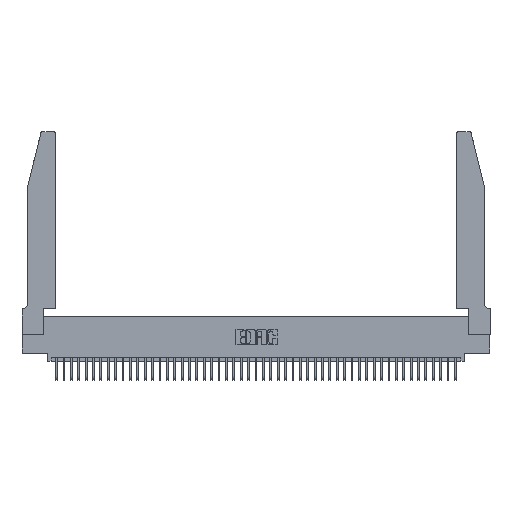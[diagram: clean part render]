
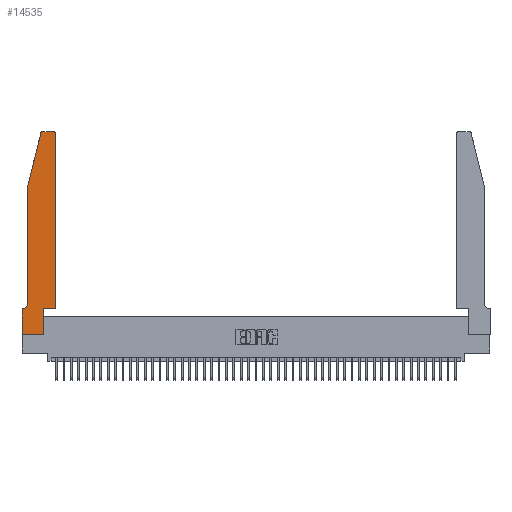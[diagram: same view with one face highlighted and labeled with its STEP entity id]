
A CAD part, top view. The second image highlights one B-rep face of the part: STEP entity #14535.
In plain terms, the highlighted planar face has unit normal (0, 0, 1).
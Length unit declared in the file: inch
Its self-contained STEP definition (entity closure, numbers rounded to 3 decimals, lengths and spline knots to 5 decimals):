
#66 = CARTESIAN_POINT ( 'NONE',  ( 0.2865, 0.35, 0.37 ) ) ;
#207 = VECTOR ( 'NONE', #40731, 39.37008 ) ;
#488 = CARTESIAN_POINT ( 'NONE',  ( 0., 0., 0.37 ) ) ;
#672 = CARTESIAN_POINT ( 'NONE',  ( 0.25487, 2.72718, 0.37 ) ) ;
#679 = VERTEX_POINT ( 'NONE', #22662 ) ;
#1018 = CARTESIAN_POINT ( 'NONE',  ( 0.4505, 0.35, 0.37 ) ) ;
#1709 = ORIENTED_EDGE ( 'NONE', *, *, #38244, .T. ) ;
#1734 = VECTOR ( 'NONE', #15758, 39.37008 ) ;
#2742 = DIRECTION ( 'NONE',  ( 0., 0., -1. ) ) ;
#3616 = CARTESIAN_POINT ( 'NONE',  ( 0.4505, 2.72, 0.37 ) ) ;
#4556 = DIRECTION ( 'NONE',  ( 1., 0., 0. ) ) ;
#5175 = ORIENTED_EDGE ( 'NONE', *, *, #9305, .T. ) ;
#5459 = LINE ( 'NONE', #34822, #13604 ) ;
#5565 = EDGE_CURVE ( 'NONE', #23691, #679, #12324, .T. ) ;
#5816 = ORIENTED_EDGE ( 'NONE', *, *, #7570, .T. ) ;
#6115 = VECTOR ( 'NONE', #41882, 39.37008 ) ;
#6336 = DIRECTION ( 'NONE',  ( 0., 0., 1. ) ) ;
#7570 = EDGE_CURVE ( 'NONE', #679, #35462, #41618, .T. ) ;
#8010 = DIRECTION ( 'NONE',  ( 0., 0., 1. ) ) ;
#8549 = VECTOR ( 'NONE', #20804, 39.37008 ) ;
#8889 = CARTESIAN_POINT ( 'NONE',  ( 0., 0., 0.37 ) ) ;
#9305 = EDGE_CURVE ( 'NONE', #35161, #23691, #12221, .T. ) ;
#9430 = VERTEX_POINT ( 'NONE', #10412 ) ;
#9630 = DIRECTION ( 'NONE',  ( -1., 0., 0. ) ) ;
#10412 = CARTESIAN_POINT ( 'NONE',  ( 0.4205, 2.75, 0.37 ) ) ;
#10415 = CIRCLE ( 'NONE', #20290, 0.03 ) ;
#10791 = EDGE_CURVE ( 'NONE', #35462, #15622, #33499, .T. ) ;
#10828 = PLANE ( 'NONE',  #28734 ) ;
#12221 = CIRCLE ( 'NONE', #22729, 0.07 ) ;
#12324 = LINE ( 'NONE', #30077, #20281 ) ;
#12416 = CARTESIAN_POINT ( 'NONE',  ( 0.0755, 2., 0.37 ) ) ;
#12684 = LINE ( 'NONE', #12416, #29736 ) ;
#13153 = VERTEX_POINT ( 'NONE', #42858 ) ;
#13346 = CARTESIAN_POINT ( 'NONE',  ( 0.0755, 2., 0.37 ) ) ;
#13604 = VECTOR ( 'NONE', #17772, 39.37008 ) ;
#13966 = CIRCLE ( 'NONE', #28498, 0.03 ) ;
#14257 = DIRECTION ( 'NONE',  ( 0., 0., 1. ) ) ;
#14535 = ADVANCED_FACE ( 'NONE', ( #36856 ), #10828, .T. ) ;
#14954 = EDGE_CURVE ( 'NONE', #28497, #17922, #13966, .T. ) ;
#15125 = ORIENTED_EDGE ( 'NONE', *, *, #26825, .T. ) ;
#15622 = VERTEX_POINT ( 'NONE', #16986 ) ;
#15758 = DIRECTION ( 'NONE',  ( 0., 1., 0. ) ) ;
#16553 = ORIENTED_EDGE ( 'NONE', *, *, #17469, .T. ) ;
#16986 = CARTESIAN_POINT ( 'NONE',  ( 0.2865, 0., 0.37 ) ) ;
#17469 = EDGE_CURVE ( 'NONE', #13153, #20278, #30271, .T. ) ;
#17772 = DIRECTION ( 'NONE',  ( -1., 0., 0. ) ) ;
#17922 = VERTEX_POINT ( 'NONE', #672 ) ;
#19281 = EDGE_CURVE ( 'NONE', #43504, #13153, #43596, .T. ) ;
#20278 = VERTEX_POINT ( 'NONE', #3616 ) ;
#20281 = VECTOR ( 'NONE', #9630, 39.37008 ) ;
#20290 = AXIS2_PLACEMENT_3D ( 'NONE', #28475, #8010, #31989 ) ;
#20804 = DIRECTION ( 'NONE',  ( 0., 1., 0. ) ) ;
#21952 = ORIENTED_EDGE ( 'NONE', *, *, #14954, .T. ) ;
#22313 = VECTOR ( 'NONE', #36286, 39.37008 ) ;
#22662 = CARTESIAN_POINT ( 'NONE',  ( 0., 0.35, 0.37 ) ) ;
#22723 = EDGE_CURVE ( 'NONE', #9430, #28497, #5459, .T. ) ;
#22729 = AXIS2_PLACEMENT_3D ( 'NONE', #23378, #2742, #26778 ) ;
#23218 = EDGE_LOOP ( 'NONE', ( #23835, #21952, #43551, #15125, #5175, #38683, #5816, #31311, #1709, #23413, #16553, #39339 ) ) ;
#23378 = CARTESIAN_POINT ( 'NONE',  ( 0.0055, 0.42, 0.37 ) ) ;
#23413 = ORIENTED_EDGE ( 'NONE', *, *, #19281, .T. ) ;
#23691 = VERTEX_POINT ( 'NONE', #37293 ) ;
#23835 = ORIENTED_EDGE ( 'NONE', *, *, #22723, .T. ) ;
#25575 = EDGE_CURVE ( 'NONE', #17922, #29035, #36844, .T. ) ;
#26284 = CARTESIAN_POINT ( 'NONE',  ( 0.284, 2.75, 0.37 ) ) ;
#26545 = CARTESIAN_POINT ( 'NONE',  ( 0., 0., 0.37 ) ) ;
#26778 = DIRECTION ( 'NONE',  ( -1., 0., 0. ) ) ;
#26825 = EDGE_CURVE ( 'NONE', #29035, #35161, #12684, .T. ) ;
#26830 = CARTESIAN_POINT ( 'NONE',  ( 0.284, 2.72, 0.37 ) ) ;
#26833 = CARTESIAN_POINT ( 'NONE',  ( 0.0755, 2., 0.37 ) ) ;
#27778 = CARTESIAN_POINT ( 'NONE',  ( 0., 0.35, 0.37 ) ) ;
#28475 = CARTESIAN_POINT ( 'NONE',  ( 0.4205, 2.72, 0.37 ) ) ;
#28497 = VERTEX_POINT ( 'NONE', #26284 ) ;
#28498 = AXIS2_PLACEMENT_3D ( 'NONE', #26830, #6336, #30309 ) ;
#28734 = AXIS2_PLACEMENT_3D ( 'NONE', #27778, #14257, #38201 ) ;
#29035 = VERTEX_POINT ( 'NONE', #26833 ) ;
#29358 = DIRECTION ( 'NONE',  ( 0., -1., 0. ) ) ;
#29736 = VECTOR ( 'NONE', #29358, 39.37008 ) ;
#30077 = CARTESIAN_POINT ( 'NONE',  ( 0.0755, 0.35, 0.37 ) ) ;
#30271 = LINE ( 'NONE', #32807, #1734 ) ;
#30309 = DIRECTION ( 'NONE',  ( 1., 0., 0. ) ) ;
#31311 = ORIENTED_EDGE ( 'NONE', *, *, #10791, .T. ) ;
#31989 = DIRECTION ( 'NONE',  ( 1., 0., 0. ) ) ;
#32807 = CARTESIAN_POINT ( 'NONE',  ( 0.4505, 0.35, 0.37 ) ) ;
#33499 = LINE ( 'NONE', #488, #6115 ) ;
#34822 = CARTESIAN_POINT ( 'NONE',  ( 0.2605, 2.75, 0.37 ) ) ;
#35161 = VERTEX_POINT ( 'NONE', #38807 ) ;
#35309 = CARTESIAN_POINT ( 'NONE',  ( 0.2865, 0.35, 0.37 ) ) ;
#35462 = VERTEX_POINT ( 'NONE', #26545 ) ;
#36286 = DIRECTION ( 'NONE',  ( 0., -1., 0. ) ) ;
#36628 = VECTOR ( 'NONE', #4556, 39.37008 ) ;
#36844 = LINE ( 'NONE', #13346, #207 ) ;
#36856 = FACE_OUTER_BOUND ( 'NONE', #23218, .T. ) ;
#37293 = CARTESIAN_POINT ( 'NONE',  ( 0.0055, 0.35, 0.37 ) ) ;
#38201 = DIRECTION ( 'NONE',  ( 1., 0., 0. ) ) ;
#38244 = EDGE_CURVE ( 'NONE', #15622, #43504, #43887, .T. ) ;
#38683 = ORIENTED_EDGE ( 'NONE', *, *, #5565, .T. ) ;
#38807 = CARTESIAN_POINT ( 'NONE',  ( 0.0755, 0.42, 0.37 ) ) ;
#39339 = ORIENTED_EDGE ( 'NONE', *, *, #40664, .T. ) ;
#40664 = EDGE_CURVE ( 'NONE', #20278, #9430, #10415, .T. ) ;
#40731 = DIRECTION ( 'NONE',  ( -0.239, -0.971, 0. ) ) ;
#41618 = LINE ( 'NONE', #8889, #22313 ) ;
#41882 = DIRECTION ( 'NONE',  ( 1., 0., 0. ) ) ;
#42858 = CARTESIAN_POINT ( 'NONE',  ( 0.4505, 0.35, 0.37 ) ) ;
#43504 = VERTEX_POINT ( 'NONE', #35309 ) ;
#43551 = ORIENTED_EDGE ( 'NONE', *, *, #25575, .T. ) ;
#43596 = LINE ( 'NONE', #1018, #36628 ) ;
#43887 = LINE ( 'NONE', #66, #8549 ) ;
